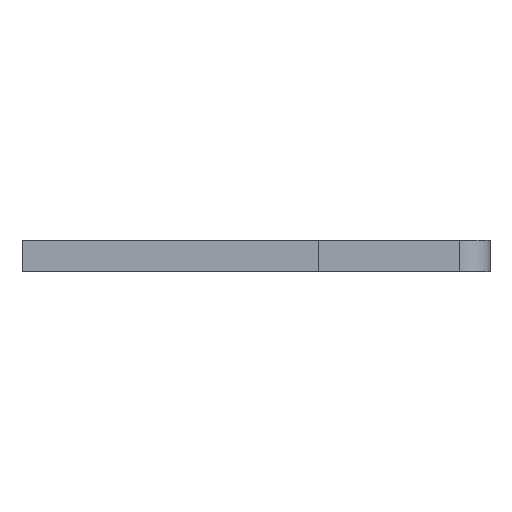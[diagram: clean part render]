
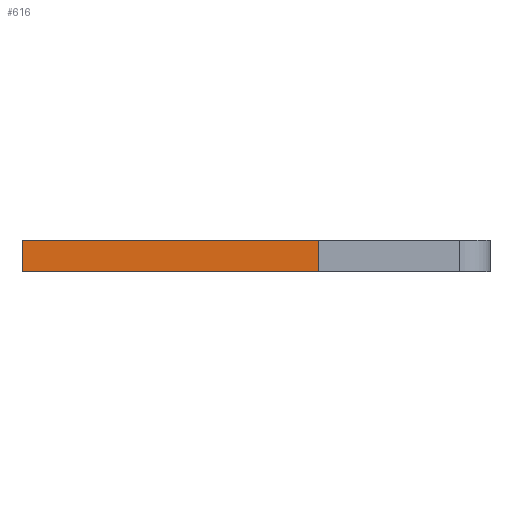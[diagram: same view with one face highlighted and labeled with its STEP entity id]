
A CAD part, left-side view. The second image highlights one B-rep face of the part: STEP entity #616.
In plain terms, the highlighted face is planar.
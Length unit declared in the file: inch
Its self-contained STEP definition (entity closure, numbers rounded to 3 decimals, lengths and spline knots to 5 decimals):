
#2 = LINE ( 'NONE', #878, #423 ) ;
#19 = CARTESIAN_POINT ( 'NONE',  ( -0.01, 0.15, -0.04 ) ) ;
#83 = ORIENTED_EDGE ( 'NONE', *, *, #1044, .F. ) ;
#101 = EDGE_LOOP ( 'NONE', ( #512, #783, #83, #474 ) ) ;
#167 = AXIS2_PLACEMENT_3D ( 'NONE', #600, #728, #345 ) ;
#179 = CARTESIAN_POINT ( 'NONE',  ( -0.01, 0.15, -0.04 ) ) ;
#203 = EDGE_CURVE ( 'NONE', #415, #801, #737, .T. ) ;
#233 = DIRECTION ( 'NONE',  ( -1., 0., 0. ) ) ;
#257 = VERTEX_POINT ( 'NONE', #712 ) ;
#295 = LINE ( 'NONE', #1025, #603 ) ;
#325 = EDGE_CURVE ( 'NONE', #363, #257, #2, .T. ) ;
#345 = DIRECTION ( 'NONE',  ( 1., 0., 0. ) ) ;
#363 = VERTEX_POINT ( 'NONE', #581 ) ;
#405 = VECTOR ( 'NONE', #471, 39.37008 ) ;
#411 = LINE ( 'NONE', #19, #644 ) ;
#415 = VERTEX_POINT ( 'NONE', #884 ) ;
#423 = VECTOR ( 'NONE', #233, 39.37008 ) ;
#427 = PLANE ( 'NONE',  #167 ) ;
#471 = DIRECTION ( 'NONE',  ( -1., 0., 0. ) ) ;
#474 = ORIENTED_EDGE ( 'NONE', *, *, #325, .T. ) ;
#512 = ORIENTED_EDGE ( 'NONE', *, *, #864, .T. ) ;
#565 = CARTESIAN_POINT ( 'NONE',  ( 0.01, 0.15, -0.04 ) ) ;
#581 = CARTESIAN_POINT ( 'NONE',  ( 0.01, -0.04, -0.04 ) ) ;
#600 = CARTESIAN_POINT ( 'NONE',  ( 0.01, 0.15, -0.04 ) ) ;
#603 = VECTOR ( 'NONE', #931, 39.37008 ) ;
#616 = ADVANCED_FACE ( 'NONE', ( #660 ), #427, .F. ) ;
#617 = DIRECTION ( 'NONE',  ( 0., 1., 0. ) ) ;
#644 = VECTOR ( 'NONE', #617, 39.37008 ) ;
#660 = FACE_OUTER_BOUND ( 'NONE', #101, .T. ) ;
#712 = CARTESIAN_POINT ( 'NONE',  ( -0.01, -0.04, -0.04 ) ) ;
#728 = DIRECTION ( 'NONE',  ( 0., 0., 1. ) ) ;
#737 = LINE ( 'NONE', #565, #405 ) ;
#783 = ORIENTED_EDGE ( 'NONE', *, *, #203, .F. ) ;
#801 = VERTEX_POINT ( 'NONE', #179 ) ;
#864 = EDGE_CURVE ( 'NONE', #257, #801, #411, .T. ) ;
#878 = CARTESIAN_POINT ( 'NONE',  ( 0.01, -0.04, -0.04 ) ) ;
#884 = CARTESIAN_POINT ( 'NONE',  ( 0.01, 0.15, -0.04 ) ) ;
#931 = DIRECTION ( 'NONE',  ( 0., 1., 0. ) ) ;
#1025 = CARTESIAN_POINT ( 'NONE',  ( 0.01, 0.15, -0.04 ) ) ;
#1044 = EDGE_CURVE ( 'NONE', #363, #415, #295, .T. ) ;
